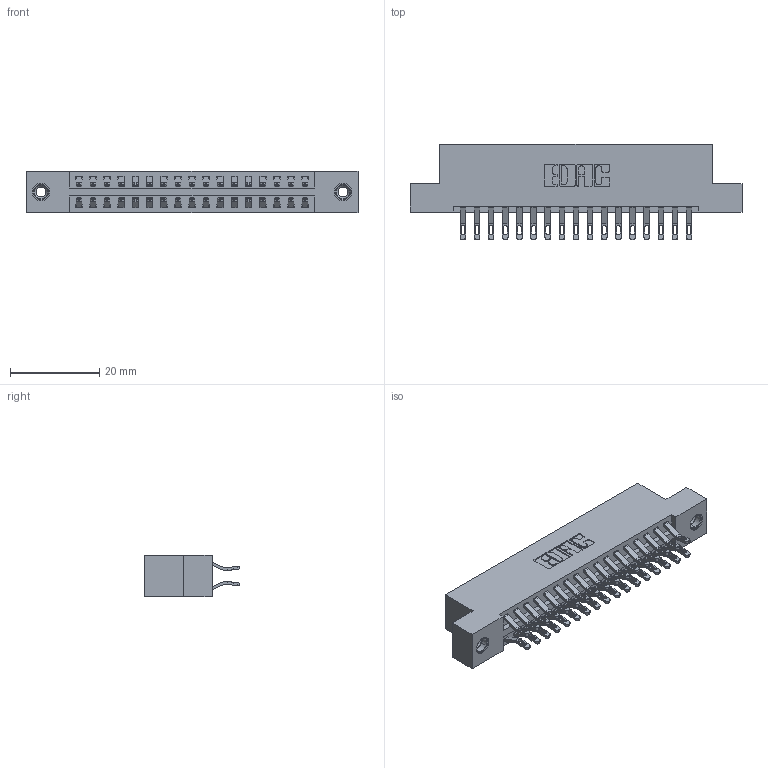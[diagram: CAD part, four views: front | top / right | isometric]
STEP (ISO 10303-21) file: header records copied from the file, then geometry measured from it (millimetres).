
FILE_DESCRIPTION (( 'STEP AP203' ), '1' );
FILE_NAME ('346-034-555-208.STEP', '2018-08-23T22:55:10', ( '' ), ( '' ), 'SwSTEP 2.0', 'SolidWorks 2016', '' );
FILE_SCHEMA (( 'CONFIG_CONTROL_DESIGN' ));
Length unit declared in the file: inch
Products named in the file (4): 346-034-555-208; 346 Part_Flush Mounting Lugs - 0.156 Dia-TI; 345-292-001_555 Tail; 345-250-001_345-250-003-102
Assembly tree (37 placements, depth 2):
  346-034-555-208
    346 Part_Flush Mounting Lugs - 0.156 Dia-TI
    345-292-001_555 Tail  x34
    345-250-001_345-250-003-102  x2
Bounding box: 74.55 x 21.46 x 9.4 mm (x, y, z)
Volume: 7167.4 mm3; surface area: 9830.7 mm2
Topology: 37 solids, 37 shells, 2154 faces, 6687 edges, 4450 vertices
Faces by surface type: plane 1230, cylinder 908, cone 12, torus 4
Entity records: 15972 total; most frequent: CARTESIAN_POINT 2685, ORIENTED_EDGE 2582, DIRECTION 2413, EDGE_CURVE 1291, VECTOR 1051, LINE 1051, VERTEX_POINT 856, AXIS2_PLACEMENT_3D 681
